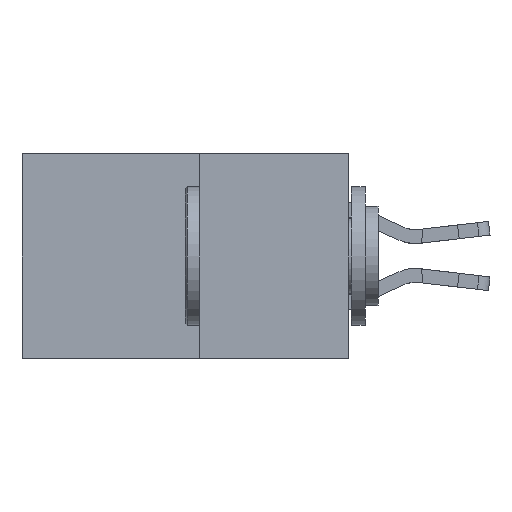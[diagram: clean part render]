
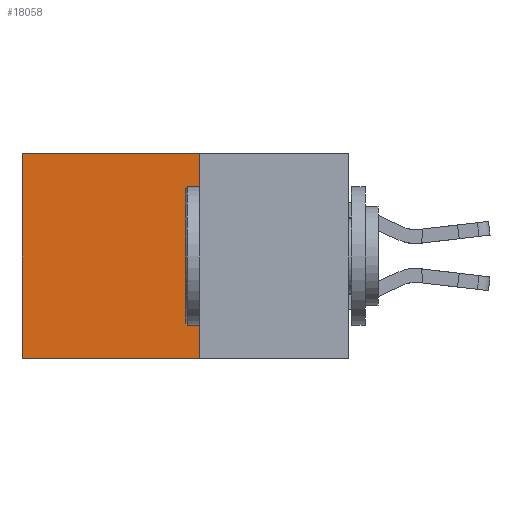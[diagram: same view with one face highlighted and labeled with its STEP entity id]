
A CAD part, left-side view. The second image highlights one B-rep face of the part: STEP entity #18058.
In plain terms, the highlighted planar face has unit normal (-1, 0, 0).
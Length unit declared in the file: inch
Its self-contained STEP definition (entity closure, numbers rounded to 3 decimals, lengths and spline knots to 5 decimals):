
#1052 = CARTESIAN_POINT ( 'NONE',  ( 0.277, 0.27, -0.37 ) ) ;
#1921 = VERTEX_POINT ( 'NONE', #23842 ) ;
#2682 = VECTOR ( 'NONE', #8227, 39.37008 ) ;
#4568 = LINE ( 'NONE', #21718, #22079 ) ;
#6894 = ORIENTED_EDGE ( 'NONE', *, *, #9361, .F. ) ;
#8213 = VERTEX_POINT ( 'NONE', #9217 ) ;
#8227 = DIRECTION ( 'NONE',  ( 0., 0., -1. ) ) ;
#8658 = VECTOR ( 'NONE', #14533, 39.37008 ) ;
#8733 = CARTESIAN_POINT ( 'NONE',  ( 0.277, 0.27, -0.37 ) ) ;
#9001 = VERTEX_POINT ( 'NONE', #28221 ) ;
#9217 = CARTESIAN_POINT ( 'NONE',  ( 0.277, 0.59, 0. ) ) ;
#9361 = EDGE_CURVE ( 'NONE', #28190, #9001, #21658, .T. ) ;
#9713 = CARTESIAN_POINT ( 'NONE',  ( 0.277, 0.27, 0. ) ) ;
#11040 = AXIS2_PLACEMENT_3D ( 'NONE', #8733, #15831, #13547 ) ;
#11128 = PLANE ( 'NONE',  #11040 ) ;
#13047 = FACE_OUTER_BOUND ( 'NONE', #23229, .T. ) ;
#13547 = DIRECTION ( 'NONE',  ( 0., 0., -1. ) ) ;
#14533 = DIRECTION ( 'NONE',  ( 0., 1., 0. ) ) ;
#14867 = LINE ( 'NONE', #22947, #15597 ) ;
#15034 = LINE ( 'NONE', #9713, #8658 ) ;
#15597 = VECTOR ( 'NONE', #18242, 39.37008 ) ;
#15831 = DIRECTION ( 'NONE',  ( 1., 0., 0. ) ) ;
#18058 = ADVANCED_FACE ( 'NONE', ( #13047 ), #11128, .F. ) ;
#18242 = DIRECTION ( 'NONE',  ( 0., 0., -1. ) ) ;
#18681 = EDGE_CURVE ( 'NONE', #8213, #1921, #14867, .T. ) ;
#21658 = LINE ( 'NONE', #1052, #2682 ) ;
#21718 = CARTESIAN_POINT ( 'NONE',  ( 0.277, 0.27, -0.37 ) ) ;
#22079 = VECTOR ( 'NONE', #24066, 39.37008 ) ;
#22947 = CARTESIAN_POINT ( 'NONE',  ( 0.277, 0.59, -0.37 ) ) ;
#23229 = EDGE_LOOP ( 'NONE', ( #28031, #24073, #6894, #29601 ) ) ;
#23842 = CARTESIAN_POINT ( 'NONE',  ( 0.277, 0.59, -0.37 ) ) ;
#24039 = EDGE_CURVE ( 'NONE', #9001, #1921, #4568, .T. ) ;
#24066 = DIRECTION ( 'NONE',  ( 0., 1., 0. ) ) ;
#24073 = ORIENTED_EDGE ( 'NONE', *, *, #24039, .F. ) ;
#24728 = EDGE_CURVE ( 'NONE', #28190, #8213, #15034, .T. ) ;
#27972 = CARTESIAN_POINT ( 'NONE',  ( 0.277, 0.27, 0. ) ) ;
#28031 = ORIENTED_EDGE ( 'NONE', *, *, #18681, .T. ) ;
#28190 = VERTEX_POINT ( 'NONE', #27972 ) ;
#28221 = CARTESIAN_POINT ( 'NONE',  ( 0.277, 0.27, -0.37 ) ) ;
#29601 = ORIENTED_EDGE ( 'NONE', *, *, #24728, .T. ) ;
